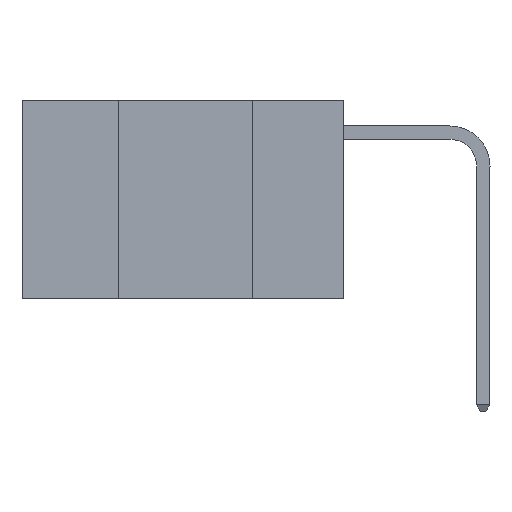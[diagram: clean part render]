
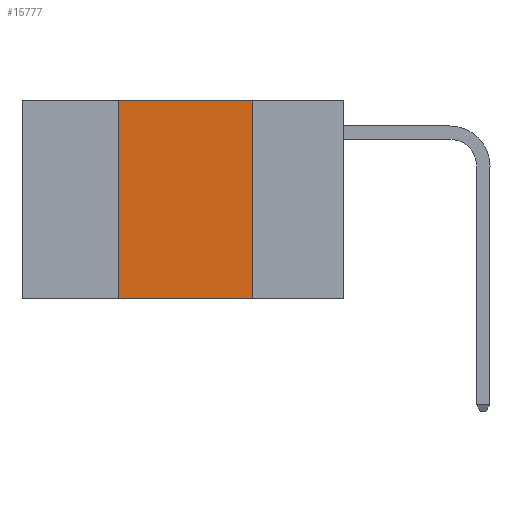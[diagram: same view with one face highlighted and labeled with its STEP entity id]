
A CAD part, left-side view. The second image highlights one B-rep face of the part: STEP entity #15777.
In plain terms, the highlighted planar face has unit normal (-1, 0, 0).
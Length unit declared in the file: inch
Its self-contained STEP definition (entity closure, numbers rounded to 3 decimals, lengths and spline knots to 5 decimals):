
#33 = VECTOR ( 'NONE', #3759, 39.37008 ) ;
#503 = ORIENTED_EDGE ( 'NONE', *, *, #7071, .F. ) ;
#733 = VECTOR ( 'NONE', #15329, 39.37008 ) ;
#1141 = EDGE_CURVE ( 'NONE', #8262, #8762, #4024, .T. ) ;
#1802 = CARTESIAN_POINT ( 'NONE',  ( 0., 0.42, 0. ) ) ;
#1810 = DIRECTION ( 'NONE',  ( 0., 0., 1. ) ) ;
#2408 = CARTESIAN_POINT ( 'NONE',  ( 0., 0.42, -0.37 ) ) ;
#2888 = EDGE_CURVE ( 'NONE', #8262, #8660, #4142, .T. ) ;
#3759 = DIRECTION ( 'NONE',  ( 0., 0., -1. ) ) ;
#3768 = EDGE_CURVE ( 'NONE', #8259, #8762, #10536, .T. ) ;
#4024 = LINE ( 'NONE', #8288, #14172 ) ;
#4142 = LINE ( 'NONE', #1802, #4554 ) ;
#4419 = DIRECTION ( 'NONE',  ( 1., 0., 0. ) ) ;
#4554 = VECTOR ( 'NONE', #1810, 39.37008 ) ;
#7071 = EDGE_CURVE ( 'NONE', #8660, #8259, #7711, .T. ) ;
#7711 = LINE ( 'NONE', #13986, #733 ) ;
#8085 = EDGE_LOOP ( 'NONE', ( #13695, #503, #14955, #8748 ) ) ;
#8259 = VERTEX_POINT ( 'NONE', #8922 ) ;
#8262 = VERTEX_POINT ( 'NONE', #2408 ) ;
#8288 = CARTESIAN_POINT ( 'NONE',  ( 0., 0.6, -0.37 ) ) ;
#8323 = DIRECTION ( 'NONE',  ( 0., -1., 0. ) ) ;
#8660 = VERTEX_POINT ( 'NONE', #12496 ) ;
#8748 = ORIENTED_EDGE ( 'NONE', *, *, #1141, .T. ) ;
#8762 = VERTEX_POINT ( 'NONE', #13315 ) ;
#8922 = CARTESIAN_POINT ( 'NONE',  ( 0., 0.17, 0. ) ) ;
#8935 = FACE_OUTER_BOUND ( 'NONE', #8085, .T. ) ;
#9029 = CARTESIAN_POINT ( 'NONE',  ( 0., 0.17, 0. ) ) ;
#9679 = CARTESIAN_POINT ( 'NONE',  ( 0., 0.6, 0. ) ) ;
#10536 = LINE ( 'NONE', #9029, #33 ) ;
#12351 = PLANE ( 'NONE',  #16619 ) ;
#12496 = CARTESIAN_POINT ( 'NONE',  ( 0., 0.42, 0. ) ) ;
#13315 = CARTESIAN_POINT ( 'NONE',  ( 0., 0.17, -0.37 ) ) ;
#13677 = DIRECTION ( 'NONE',  ( 0., 0., -1. ) ) ;
#13695 = ORIENTED_EDGE ( 'NONE', *, *, #3768, .F. ) ;
#13986 = CARTESIAN_POINT ( 'NONE',  ( 0., 0.6, 0. ) ) ;
#14172 = VECTOR ( 'NONE', #8323, 39.37008 ) ;
#14955 = ORIENTED_EDGE ( 'NONE', *, *, #2888, .F. ) ;
#15329 = DIRECTION ( 'NONE',  ( 0., -1., 0. ) ) ;
#15777 = ADVANCED_FACE ( 'NONE', ( #8935 ), #12351, .F. ) ;
#16619 = AXIS2_PLACEMENT_3D ( 'NONE', #9679, #4419, #13677 ) ;
